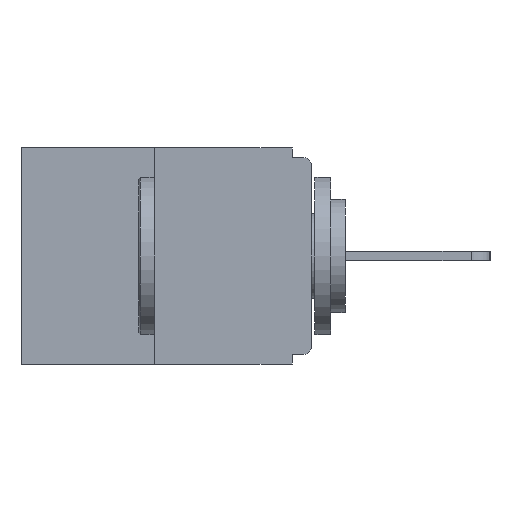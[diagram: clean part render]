
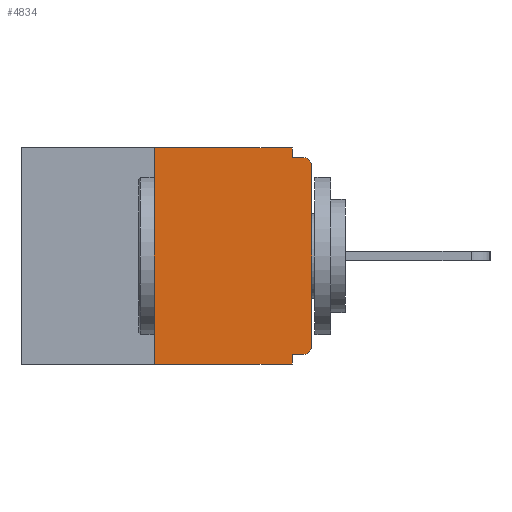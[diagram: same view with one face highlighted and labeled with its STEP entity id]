
A CAD part, left-side view. The second image highlights one B-rep face of the part: STEP entity #4834.
In plain terms, the highlighted planar face has unit normal (-1, 0, 0).
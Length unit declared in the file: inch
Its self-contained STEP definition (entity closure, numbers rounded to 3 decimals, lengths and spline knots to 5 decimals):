
#186 = CIRCLE ( 'NONE', #18416, 0.015 ) ;
#554 = LINE ( 'NONE', #14646, #12185 ) ;
#920 = EDGE_CURVE ( 'NONE', #15520, #7097, #1894, .T. ) ;
#963 = DIRECTION ( 'NONE',  ( 0., -1., 0. ) ) ;
#1469 = CARTESIAN_POINT ( 'NONE',  ( 0., 0., 0. ) ) ;
#1607 = CIRCLE ( 'NONE', #3149, 0.015 ) ;
#1891 = ORIENTED_EDGE ( 'NONE', *, *, #6326, .T. ) ;
#1894 = LINE ( 'NONE', #1469, #5504 ) ;
#3100 = LINE ( 'NONE', #14452, #7203 ) ;
#3116 = CARTESIAN_POINT ( 'NONE',  ( 0., 0.031, 0. ) ) ;
#3149 = AXIS2_PLACEMENT_3D ( 'NONE', #13248, #4219, #14827 ) ;
#3345 = VERTEX_POINT ( 'NONE', #5202 ) ;
#3474 = VERTEX_POINT ( 'NONE', #6960 ) ;
#3970 = DIRECTION ( 'NONE',  ( -1., 0., 0. ) ) ;
#4219 = DIRECTION ( 'NONE',  ( -1., 0., 0. ) ) ;
#4620 = LINE ( 'NONE', #7314, #12625 ) ;
#4745 = CARTESIAN_POINT ( 'NONE',  ( 0., 0., -0.03 ) ) ;
#4774 = ORIENTED_EDGE ( 'NONE', *, *, #920, .T. ) ;
#4834 = ADVANCED_FACE ( 'NONE', ( #17764 ), #10132, .F. ) ;
#5058 = CARTESIAN_POINT ( 'NONE',  ( 0., 0.031, -0.343 ) ) ;
#5202 = CARTESIAN_POINT ( 'NONE',  ( 0., 0.031, -0.015 ) ) ;
#5504 = VECTOR ( 'NONE', #12138, 39.37008 ) ;
#5598 = LINE ( 'NONE', #3116, #8701 ) ;
#5669 = CARTESIAN_POINT ( 'NONE',  ( 0., 0.46, 0. ) ) ;
#6326 = EDGE_CURVE ( 'NONE', #17054, #16420, #12062, .T. ) ;
#6417 = VERTEX_POINT ( 'NONE', #8977 ) ;
#6492 = ORIENTED_EDGE ( 'NONE', *, *, #16253, .F. ) ;
#6635 = DIRECTION ( 'NONE',  ( 0., 0., -1. ) ) ;
#6959 = CARTESIAN_POINT ( 'NONE',  ( 0., 0.031, -0.343 ) ) ;
#6960 = CARTESIAN_POINT ( 'NONE',  ( 0., 0.015, -0.015 ) ) ;
#6998 = VERTEX_POINT ( 'NONE', #7176 ) ;
#7097 = VERTEX_POINT ( 'NONE', #4745 ) ;
#7176 = CARTESIAN_POINT ( 'NONE',  ( 0., 0.015, -0.328 ) ) ;
#7203 = VECTOR ( 'NONE', #15987, 39.37008 ) ;
#7314 = CARTESIAN_POINT ( 'NONE',  ( 0., 0.25, 0. ) ) ;
#8562 = VECTOR ( 'NONE', #18809, 39.37008 ) ;
#8701 = VECTOR ( 'NONE', #12102, 39.37008 ) ;
#8853 = ORIENTED_EDGE ( 'NONE', *, *, #11025, .T. ) ;
#8977 = CARTESIAN_POINT ( 'NONE',  ( 0., 0.031, -0.328 ) ) ;
#9421 = DIRECTION ( 'NONE',  ( 0., 0., -1. ) ) ;
#9657 = EDGE_CURVE ( 'NONE', #13059, #13355, #3100, .T. ) ;
#9846 = LINE ( 'NONE', #5058, #17371 ) ;
#9877 = CARTESIAN_POINT ( 'NONE',  ( 0., 0., -0.328 ) ) ;
#10002 = CARTESIAN_POINT ( 'NONE',  ( 0., 0.46, -0.343 ) ) ;
#10132 = PLANE ( 'NONE',  #14525 ) ;
#10252 = ORIENTED_EDGE ( 'NONE', *, *, #16068, .F. ) ;
#10268 = EDGE_CURVE ( 'NONE', #6998, #15520, #186, .T. ) ;
#10350 = DIRECTION ( 'NONE',  ( 0., -1., 0. ) ) ;
#10460 = ORIENTED_EDGE ( 'NONE', *, *, #10860, .F. ) ;
#10860 = EDGE_CURVE ( 'NONE', #6998, #6417, #17035, .T. ) ;
#11025 = EDGE_CURVE ( 'NONE', #7097, #3474, #1607, .T. ) ;
#12062 = LINE ( 'NONE', #10002, #13001 ) ;
#12102 = DIRECTION ( 'NONE',  ( 0., 0., -1. ) ) ;
#12138 = DIRECTION ( 'NONE',  ( 0., 0., 1. ) ) ;
#12185 = VECTOR ( 'NONE', #963, 39.37008 ) ;
#12625 = VECTOR ( 'NONE', #17801, 39.37008 ) ;
#12785 = ORIENTED_EDGE ( 'NONE', *, *, #15638, .F. ) ;
#12999 = CARTESIAN_POINT ( 'NONE',  ( 0., 0.015, -0.313 ) ) ;
#13001 = VECTOR ( 'NONE', #10350, 39.37008 ) ;
#13011 = ORIENTED_EDGE ( 'NONE', *, *, #9657, .F. ) ;
#13059 = VERTEX_POINT ( 'NONE', #17279 ) ;
#13248 = CARTESIAN_POINT ( 'NONE',  ( 0., 0.015, -0.03 ) ) ;
#13355 = VERTEX_POINT ( 'NONE', #19270 ) ;
#14392 = CARTESIAN_POINT ( 'NONE',  ( 0., 0., -0.313 ) ) ;
#14452 = CARTESIAN_POINT ( 'NONE',  ( 0., 0.46, 0. ) ) ;
#14525 = AXIS2_PLACEMENT_3D ( 'NONE', #5669, #16568, #9421 ) ;
#14589 = DIRECTION ( 'NONE',  ( 0., 0., -1. ) ) ;
#14646 = CARTESIAN_POINT ( 'NONE',  ( 0., 0., -0.015 ) ) ;
#14827 = DIRECTION ( 'NONE',  ( 0., 0., -1. ) ) ;
#15063 = EDGE_LOOP ( 'NONE', ( #13011, #17515, #1891, #6492, #10460, #19306, #4774, #8853, #12785, #10252 ) ) ;
#15520 = VERTEX_POINT ( 'NONE', #14392 ) ;
#15638 = EDGE_CURVE ( 'NONE', #3345, #3474, #554, .T. ) ;
#15987 = DIRECTION ( 'NONE',  ( 0., -1., 0. ) ) ;
#16068 = EDGE_CURVE ( 'NONE', #13355, #3345, #5598, .T. ) ;
#16253 = EDGE_CURVE ( 'NONE', #6417, #16420, #9846, .T. ) ;
#16420 = VERTEX_POINT ( 'NONE', #6959 ) ;
#16568 = DIRECTION ( 'NONE',  ( 1., 0., 0. ) ) ;
#17035 = LINE ( 'NONE', #9877, #8562 ) ;
#17054 = VERTEX_POINT ( 'NONE', #18936 ) ;
#17156 = EDGE_CURVE ( 'NONE', #17054, #13059, #4620, .T. ) ;
#17279 = CARTESIAN_POINT ( 'NONE',  ( 0., 0.25, 0. ) ) ;
#17371 = VECTOR ( 'NONE', #6635, 39.37008 ) ;
#17515 = ORIENTED_EDGE ( 'NONE', *, *, #17156, .F. ) ;
#17764 = FACE_OUTER_BOUND ( 'NONE', #15063, .T. ) ;
#17801 = DIRECTION ( 'NONE',  ( 0., 0., 1. ) ) ;
#18416 = AXIS2_PLACEMENT_3D ( 'NONE', #12999, #3970, #14589 ) ;
#18809 = DIRECTION ( 'NONE',  ( 0., 1., 0. ) ) ;
#18936 = CARTESIAN_POINT ( 'NONE',  ( 0., 0.25, -0.343 ) ) ;
#19270 = CARTESIAN_POINT ( 'NONE',  ( 0., 0.031, 0. ) ) ;
#19306 = ORIENTED_EDGE ( 'NONE', *, *, #10268, .T. ) ;
